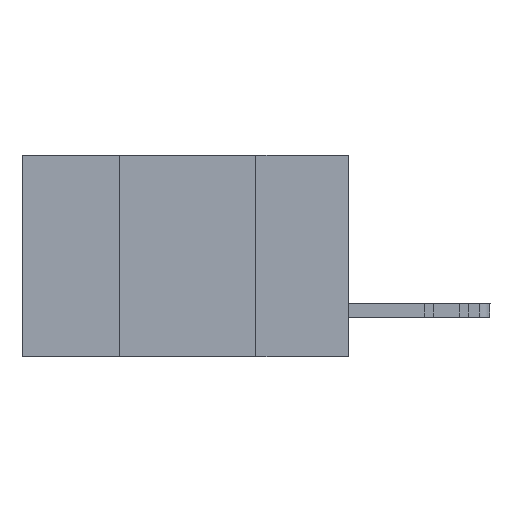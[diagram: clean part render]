
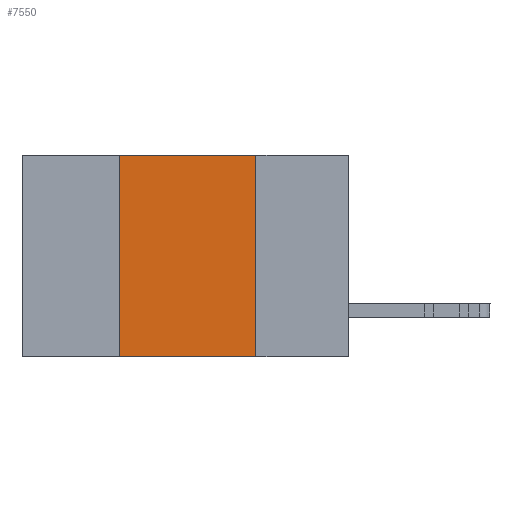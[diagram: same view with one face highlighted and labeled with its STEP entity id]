
A CAD part, left-side view. The second image highlights one B-rep face of the part: STEP entity #7550.
In plain terms, the highlighted planar face has unit normal (-1, 0, 0).
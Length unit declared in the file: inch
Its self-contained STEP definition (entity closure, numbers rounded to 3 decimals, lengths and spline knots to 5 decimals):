
#95 = CARTESIAN_POINT ( 'NONE',  ( 0., 0.42, -0.37 ) ) ;
#978 = CARTESIAN_POINT ( 'NONE',  ( 0., 0.17, -0.37 ) ) ;
#1207 = VECTOR ( 'NONE', #2930, 39.37008 ) ;
#1271 = ORIENTED_EDGE ( 'NONE', *, *, #20027, .F. ) ;
#1507 = VERTEX_POINT ( 'NONE', #16503 ) ;
#2930 = DIRECTION ( 'NONE',  ( 0., 0., -1. ) ) ;
#3585 = LINE ( 'NONE', #4665, #23122 ) ;
#4665 = CARTESIAN_POINT ( 'NONE',  ( 0., 0.42, -0.37 ) ) ;
#5225 = ORIENTED_EDGE ( 'NONE', *, *, #15343, .F. ) ;
#5604 = VERTEX_POINT ( 'NONE', #20130 ) ;
#6245 = LINE ( 'NONE', #14618, #10725 ) ;
#6419 = ORIENTED_EDGE ( 'NONE', *, *, #12096, .T. ) ;
#7550 = ADVANCED_FACE ( 'NONE', ( #8196 ), #17467, .F. ) ;
#8196 = FACE_OUTER_BOUND ( 'NONE', #12321, .T. ) ;
#9242 = VERTEX_POINT ( 'NONE', #15648 ) ;
#10014 = CARTESIAN_POINT ( 'NONE',  ( 0., 0.6, 0. ) ) ;
#10725 = VECTOR ( 'NONE', #12788, 39.37008 ) ;
#11457 = LINE ( 'NONE', #978, #1207 ) ;
#11972 = DIRECTION ( 'NONE',  ( 0., -1., 0. ) ) ;
#12096 = EDGE_CURVE ( 'NONE', #15268, #9242, #6245, .T. ) ;
#12321 = EDGE_LOOP ( 'NONE', ( #19737, #5225, #1271, #6419 ) ) ;
#12788 = DIRECTION ( 'NONE',  ( 0., -1., 0. ) ) ;
#14471 = LINE ( 'NONE', #10014, #24336 ) ;
#14618 = CARTESIAN_POINT ( 'NONE',  ( 0., 0.6, -0.37 ) ) ;
#15268 = VERTEX_POINT ( 'NONE', #95 ) ;
#15343 = EDGE_CURVE ( 'NONE', #5604, #1507, #14471, .T. ) ;
#15648 = CARTESIAN_POINT ( 'NONE',  ( 0., 0.17, -0.37 ) ) ;
#16503 = CARTESIAN_POINT ( 'NONE',  ( 0., 0.17, 0. ) ) ;
#17420 = DIRECTION ( 'NONE',  ( 1., 0., 0. ) ) ;
#17438 = CARTESIAN_POINT ( 'NONE',  ( 0., 0.6, 0. ) ) ;
#17467 = PLANE ( 'NONE',  #23740 ) ;
#17684 = DIRECTION ( 'NONE',  ( 0., 0., -1. ) ) ;
#18833 = EDGE_CURVE ( 'NONE', #1507, #9242, #11457, .T. ) ;
#19737 = ORIENTED_EDGE ( 'NONE', *, *, #18833, .F. ) ;
#19824 = DIRECTION ( 'NONE',  ( 0., 0., 1. ) ) ;
#20027 = EDGE_CURVE ( 'NONE', #15268, #5604, #3585, .T. ) ;
#20130 = CARTESIAN_POINT ( 'NONE',  ( 0., 0.42, 0. ) ) ;
#23122 = VECTOR ( 'NONE', #19824, 39.37008 ) ;
#23740 = AXIS2_PLACEMENT_3D ( 'NONE', #17438, #17420, #17684 ) ;
#24336 = VECTOR ( 'NONE', #11972, 39.37008 ) ;
